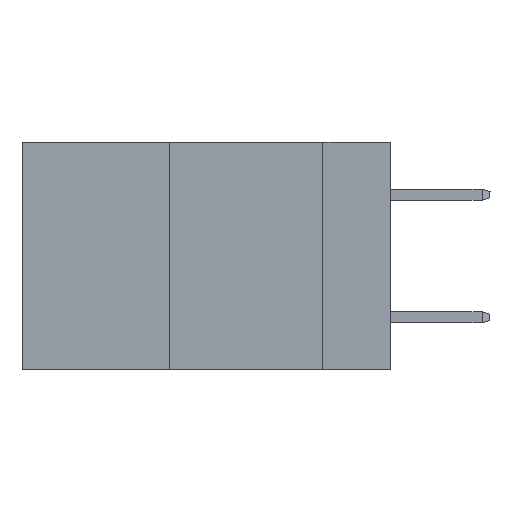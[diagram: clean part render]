
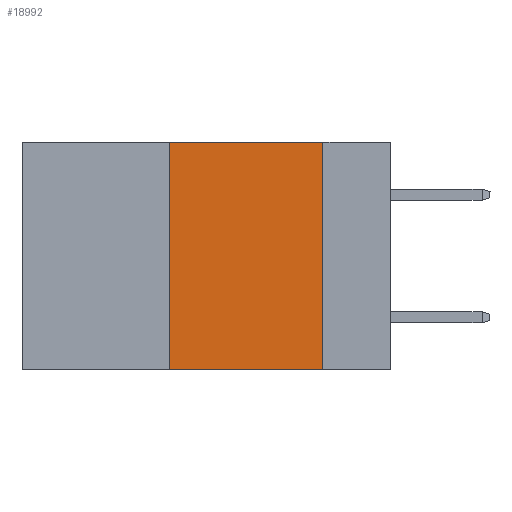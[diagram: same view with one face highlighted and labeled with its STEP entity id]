
A CAD part, left-side view. The second image highlights one B-rep face of the part: STEP entity #18992.
In plain terms, the highlighted planar face has unit normal (-1, 0, 0).
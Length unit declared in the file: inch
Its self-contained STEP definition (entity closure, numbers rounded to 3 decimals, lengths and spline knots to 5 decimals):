
#445 = CARTESIAN_POINT ( 'NONE',  ( 0., 0.36, -0.37 ) ) ;
#495 = LINE ( 'NONE', #21683, #21525 ) ;
#839 = CARTESIAN_POINT ( 'NONE',  ( 0., 0.6, 0. ) ) ;
#906 = DIRECTION ( 'NONE',  ( 0., 0., -1. ) ) ;
#1337 = DIRECTION ( 'NONE',  ( 1., 0., 0. ) ) ;
#1620 = ORIENTED_EDGE ( 'NONE', *, *, #7335, .F. ) ;
#1754 = ORIENTED_EDGE ( 'NONE', *, *, #8149, .T. ) ;
#1968 = VERTEX_POINT ( 'NONE', #2885 ) ;
#2005 = CARTESIAN_POINT ( 'NONE',  ( 0., 0.36, 0. ) ) ;
#2885 = CARTESIAN_POINT ( 'NONE',  ( 0., 0.36, 0. ) ) ;
#3683 = EDGE_CURVE ( 'NONE', #1968, #5840, #14419, .T. ) ;
#5421 = LINE ( 'NONE', #2005, #10068 ) ;
#5840 = VERTEX_POINT ( 'NONE', #14035 ) ;
#6907 = AXIS2_PLACEMENT_3D ( 'NONE', #14778, #1337, #9988 ) ;
#7263 = VECTOR ( 'NONE', #10999, 39.37008 ) ;
#7311 = CARTESIAN_POINT ( 'NONE',  ( 0., 0.11, -0.37 ) ) ;
#7335 = EDGE_CURVE ( 'NONE', #5840, #14254, #495, .T. ) ;
#8149 = EDGE_CURVE ( 'NONE', #20972, #14254, #19261, .T. ) ;
#8867 = DIRECTION ( 'NONE',  ( 0., -1., 0. ) ) ;
#9988 = DIRECTION ( 'NONE',  ( 0., 0., -1. ) ) ;
#10068 = VECTOR ( 'NONE', #14200, 39.37008 ) ;
#10999 = DIRECTION ( 'NONE',  ( 0., -1., 0. ) ) ;
#11681 = EDGE_LOOP ( 'NONE', ( #1620, #18582, #19456, #1754 ) ) ;
#13081 = PLANE ( 'NONE',  #6907 ) ;
#13157 = VECTOR ( 'NONE', #8867, 39.37008 ) ;
#14035 = CARTESIAN_POINT ( 'NONE',  ( 0., 0.11, 0. ) ) ;
#14200 = DIRECTION ( 'NONE',  ( 0., 0., 1. ) ) ;
#14254 = VERTEX_POINT ( 'NONE', #7311 ) ;
#14419 = LINE ( 'NONE', #839, #7263 ) ;
#14778 = CARTESIAN_POINT ( 'NONE',  ( 0., 0.6, 0. ) ) ;
#15821 = CARTESIAN_POINT ( 'NONE',  ( 0., 0.6, -0.37 ) ) ;
#15993 = EDGE_CURVE ( 'NONE', #20972, #1968, #5421, .T. ) ;
#18582 = ORIENTED_EDGE ( 'NONE', *, *, #3683, .F. ) ;
#18674 = FACE_OUTER_BOUND ( 'NONE', #11681, .T. ) ;
#18992 = ADVANCED_FACE ( 'NONE', ( #18674 ), #13081, .F. ) ;
#19261 = LINE ( 'NONE', #15821, #13157 ) ;
#19456 = ORIENTED_EDGE ( 'NONE', *, *, #15993, .F. ) ;
#20972 = VERTEX_POINT ( 'NONE', #445 ) ;
#21525 = VECTOR ( 'NONE', #906, 39.37008 ) ;
#21683 = CARTESIAN_POINT ( 'NONE',  ( 0., 0.11, 0. ) ) ;
